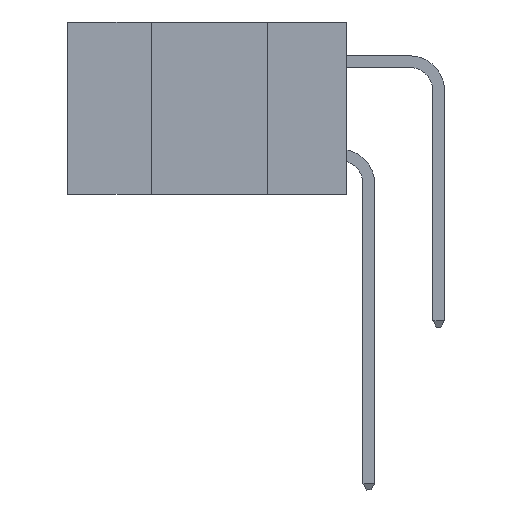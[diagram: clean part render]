
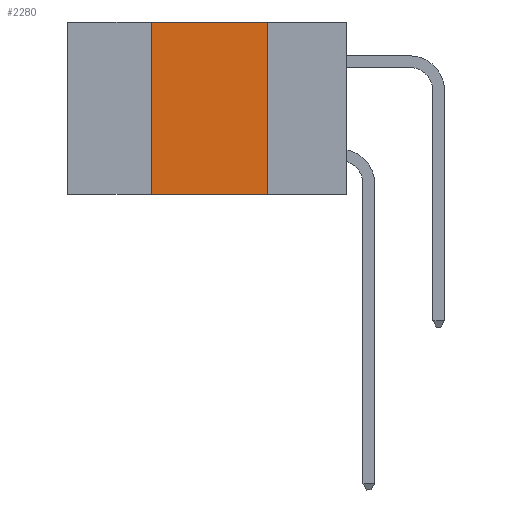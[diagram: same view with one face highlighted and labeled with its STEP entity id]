
A CAD part, left-side view. The second image highlights one B-rep face of the part: STEP entity #2280.
In plain terms, the highlighted planar face has unit normal (-1, 0, 0).
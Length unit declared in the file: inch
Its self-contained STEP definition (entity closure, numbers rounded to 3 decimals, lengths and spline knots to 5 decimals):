
#821 = CARTESIAN_POINT ( 'NONE',  ( 0., 0.17, -0.37 ) ) ;
#880 = ORIENTED_EDGE ( 'NONE', *, *, #10164, .F. ) ;
#887 = VECTOR ( 'NONE', #3077, 39.37008 ) ;
#953 = CARTESIAN_POINT ( 'NONE',  ( 0., 0.6, -0.37 ) ) ;
#1051 = CARTESIAN_POINT ( 'NONE',  ( 0., 0.17, 0. ) ) ;
#1306 = VERTEX_POINT ( 'NONE', #8366 ) ;
#1387 = CARTESIAN_POINT ( 'NONE',  ( 0., 0.42, -0.37 ) ) ;
#1819 = ORIENTED_EDGE ( 'NONE', *, *, #3162, .F. ) ;
#2037 = CARTESIAN_POINT ( 'NONE',  ( 0., 0.6, 0. ) ) ;
#2280 = ADVANCED_FACE ( 'NONE', ( #6783 ), #10830, .F. ) ;
#2522 = ORIENTED_EDGE ( 'NONE', *, *, #5892, .T. ) ;
#2827 = CARTESIAN_POINT ( 'NONE',  ( 0., 0.42, 0. ) ) ;
#2865 = VECTOR ( 'NONE', #3015, 39.37008 ) ;
#2913 = VECTOR ( 'NONE', #5196, 39.37008 ) ;
#3003 = DIRECTION ( 'NONE',  ( 0., -1., 0. ) ) ;
#3015 = DIRECTION ( 'NONE',  ( 0., -1., 0. ) ) ;
#3077 = DIRECTION ( 'NONE',  ( 0., 0., -1. ) ) ;
#3162 = EDGE_CURVE ( 'NONE', #6251, #9944, #3698, .T. ) ;
#3596 = AXIS2_PLACEMENT_3D ( 'NONE', #10883, #10790, #10778 ) ;
#3698 = LINE ( 'NONE', #5250, #2913 ) ;
#4971 = VERTEX_POINT ( 'NONE', #821 ) ;
#5196 = DIRECTION ( 'NONE',  ( 0., 0., 1. ) ) ;
#5250 = CARTESIAN_POINT ( 'NONE',  ( 0., 0.42, 0. ) ) ;
#5361 = LINE ( 'NONE', #953, #2865 ) ;
#5892 = EDGE_CURVE ( 'NONE', #6251, #4971, #5361, .T. ) ;
#6251 = VERTEX_POINT ( 'NONE', #1387 ) ;
#6783 = FACE_OUTER_BOUND ( 'NONE', #8060, .T. ) ;
#6797 = EDGE_CURVE ( 'NONE', #9944, #1306, #6972, .T. ) ;
#6972 = LINE ( 'NONE', #2037, #11020 ) ;
#8019 = LINE ( 'NONE', #1051, #887 ) ;
#8060 = EDGE_LOOP ( 'NONE', ( #880, #9142, #1819, #2522 ) ) ;
#8366 = CARTESIAN_POINT ( 'NONE',  ( 0., 0.17, 0. ) ) ;
#9142 = ORIENTED_EDGE ( 'NONE', *, *, #6797, .F. ) ;
#9944 = VERTEX_POINT ( 'NONE', #2827 ) ;
#10164 = EDGE_CURVE ( 'NONE', #1306, #4971, #8019, .T. ) ;
#10778 = DIRECTION ( 'NONE',  ( 0., 0., -1. ) ) ;
#10790 = DIRECTION ( 'NONE',  ( 1., 0., 0. ) ) ;
#10830 = PLANE ( 'NONE',  #3596 ) ;
#10883 = CARTESIAN_POINT ( 'NONE',  ( 0., 0.6, 0. ) ) ;
#11020 = VECTOR ( 'NONE', #3003, 39.37008 ) ;
